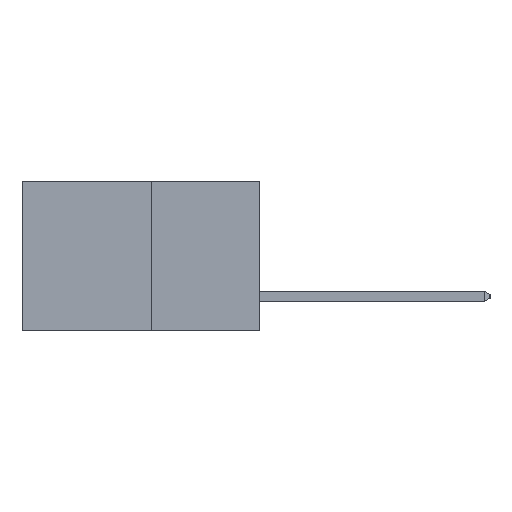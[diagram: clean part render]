
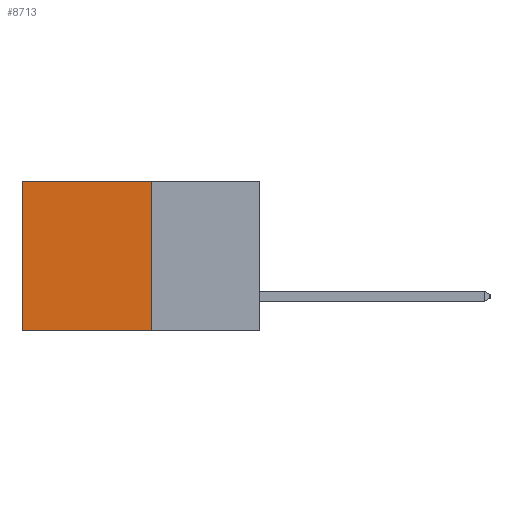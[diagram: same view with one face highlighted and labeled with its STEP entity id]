
A CAD part, left-side view. The second image highlights one B-rep face of the part: STEP entity #8713.
In plain terms, the highlighted planar face has unit normal (-1, 0, 0).
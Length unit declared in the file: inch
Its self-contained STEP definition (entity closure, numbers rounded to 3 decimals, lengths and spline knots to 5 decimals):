
#64 = DIRECTION ( 'NONE',  ( 1., 0., 0. ) ) ;
#71 = CARTESIAN_POINT ( 'NONE',  ( 0.277, 0.27, 0. ) ) ;
#685 = LINE ( 'NONE', #2760, #3357 ) ;
#1101 = CARTESIAN_POINT ( 'NONE',  ( 0.277, 0.27, -0.37 ) ) ;
#1356 = EDGE_CURVE ( 'NONE', #8047, #10290, #7102, .T. ) ;
#1735 = CARTESIAN_POINT ( 'NONE',  ( 0.277, 0.59, -0.37 ) ) ;
#2760 = CARTESIAN_POINT ( 'NONE',  ( 0.277, 0.59, -0.37 ) ) ;
#3264 = CARTESIAN_POINT ( 'NONE',  ( 0.277, 0.27, -0.37 ) ) ;
#3357 = VECTOR ( 'NONE', #10870, 39.37008 ) ;
#3602 = EDGE_LOOP ( 'NONE', ( #3954, #11503, #11745, #6556 ) ) ;
#3954 = ORIENTED_EDGE ( 'NONE', *, *, #7683, .T. ) ;
#4067 = EDGE_CURVE ( 'NONE', #13153, #5392, #8167, .T. ) ;
#4837 = VECTOR ( 'NONE', #11647, 39.37008 ) ;
#5392 = VERTEX_POINT ( 'NONE', #9307 ) ;
#6530 = AXIS2_PLACEMENT_3D ( 'NONE', #1101, #64, #7515 ) ;
#6556 = ORIENTED_EDGE ( 'NONE', *, *, #4067, .T. ) ;
#7102 = LINE ( 'NONE', #3264, #11973 ) ;
#7448 = CARTESIAN_POINT ( 'NONE',  ( 0.277, 0.27, -0.37 ) ) ;
#7515 = DIRECTION ( 'NONE',  ( 0., 0., -1. ) ) ;
#7683 = EDGE_CURVE ( 'NONE', #5392, #10290, #685, .T. ) ;
#7854 = CARTESIAN_POINT ( 'NONE',  ( 0.277, 0.27, 0. ) ) ;
#8047 = VERTEX_POINT ( 'NONE', #7448 ) ;
#8167 = LINE ( 'NONE', #71, #13033 ) ;
#8233 = EDGE_CURVE ( 'NONE', #13153, #8047, #12403, .T. ) ;
#8713 = ADVANCED_FACE ( 'NONE', ( #10119 ), #12381, .F. ) ;
#9307 = CARTESIAN_POINT ( 'NONE',  ( 0.277, 0.59, 0. ) ) ;
#10059 = DIRECTION ( 'NONE',  ( 0., 1., 0. ) ) ;
#10119 = FACE_OUTER_BOUND ( 'NONE', #3602, .T. ) ;
#10290 = VERTEX_POINT ( 'NONE', #1735 ) ;
#10686 = CARTESIAN_POINT ( 'NONE',  ( 0.277, 0.27, -0.37 ) ) ;
#10870 = DIRECTION ( 'NONE',  ( 0., 0., -1. ) ) ;
#11503 = ORIENTED_EDGE ( 'NONE', *, *, #1356, .F. ) ;
#11647 = DIRECTION ( 'NONE',  ( 0., 0., -1. ) ) ;
#11745 = ORIENTED_EDGE ( 'NONE', *, *, #8233, .F. ) ;
#11973 = VECTOR ( 'NONE', #10059, 39.37008 ) ;
#12381 = PLANE ( 'NONE',  #6530 ) ;
#12403 = LINE ( 'NONE', #10686, #4837 ) ;
#13033 = VECTOR ( 'NONE', #13272, 39.37008 ) ;
#13153 = VERTEX_POINT ( 'NONE', #7854 ) ;
#13272 = DIRECTION ( 'NONE',  ( 0., 1., 0. ) ) ;
